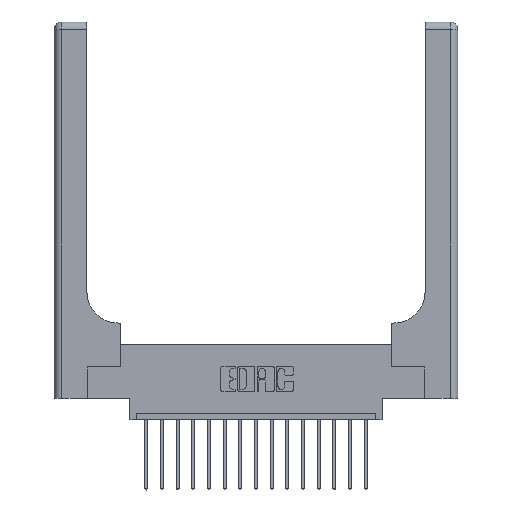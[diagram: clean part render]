
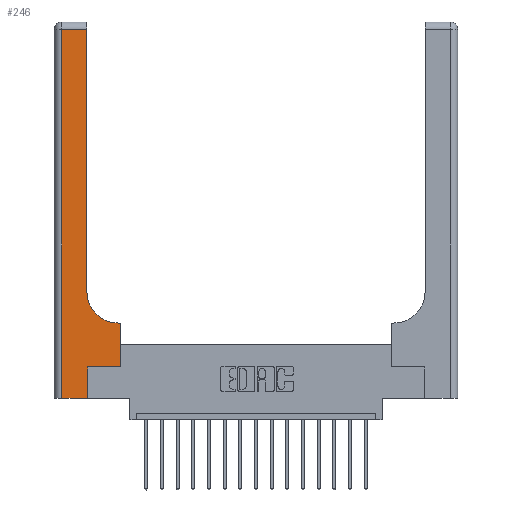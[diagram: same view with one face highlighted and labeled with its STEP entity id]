
A CAD part, top view. The second image highlights one B-rep face of the part: STEP entity #246.
In plain terms, the highlighted planar face has unit normal (0, 0, 1).
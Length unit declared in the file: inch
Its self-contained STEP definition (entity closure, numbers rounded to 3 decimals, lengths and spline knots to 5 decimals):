
#37 = EDGE_CURVE ( 'NONE', #4629, #17477, #10298, .T. ) ;
#77 = CARTESIAN_POINT ( 'NONE',  ( 0.06, 2.94, 0.37 ) ) ;
#246 = ADVANCED_FACE ( 'NONE', ( #18050 ), #10659, .F. ) ;
#384 = LINE ( 'NONE', #11235, #7409 ) ;
#398 = EDGE_CURVE ( 'NONE', #8279, #960, #17597, .T. ) ;
#650 = ORIENTED_EDGE ( 'NONE', *, *, #14773, .T. ) ;
#960 = VERTEX_POINT ( 'NONE', #5945 ) ;
#1144 = ORIENTED_EDGE ( 'NONE', *, *, #8607, .T. ) ;
#1529 = ORIENTED_EDGE ( 'NONE', *, *, #4312, .T. ) ;
#1647 = EDGE_LOOP ( 'NONE', ( #7086, #5595, #650, #1529, #4267, #12832, #17569, #1144, #8516 ) ) ;
#2311 = EDGE_CURVE ( 'NONE', #960, #9440, #13339, .T. ) ;
#2973 = LINE ( 'NONE', #3149, #10455 ) ;
#3149 = CARTESIAN_POINT ( 'NONE',  ( 0.265, 0., 0.37 ) ) ;
#3877 = LINE ( 'NONE', #10485, #13380 ) ;
#3951 = VERTEX_POINT ( 'NONE', #11939 ) ;
#4010 = AXIS2_PLACEMENT_3D ( 'NONE', #13622, #5151, #6574 ) ;
#4267 = ORIENTED_EDGE ( 'NONE', *, *, #10204, .T. ) ;
#4312 = EDGE_CURVE ( 'NONE', #15578, #3951, #3877, .T. ) ;
#4565 = CARTESIAN_POINT ( 'NONE',  ( 0.06, 3., 0.37 ) ) ;
#4629 = VERTEX_POINT ( 'NONE', #11442 ) ;
#4823 = EDGE_CURVE ( 'NONE', #9440, #11224, #384, .T. ) ;
#4839 = VECTOR ( 'NONE', #8584, 39.37008 ) ;
#5151 = DIRECTION ( 'NONE',  ( 0., 0., -1. ) ) ;
#5229 = EDGE_CURVE ( 'NONE', #17477, #16236, #8710, .T. ) ;
#5246 = CARTESIAN_POINT ( 'NONE',  ( 0.528, 0.25, 0.37 ) ) ;
#5595 = ORIENTED_EDGE ( 'NONE', *, *, #4823, .T. ) ;
#5945 = CARTESIAN_POINT ( 'NONE',  ( 0.26, 0.85, 0.37 ) ) ;
#6333 = DIRECTION ( 'NONE',  ( -1., 0., 0. ) ) ;
#6574 = DIRECTION ( 'NONE',  ( 1., 0., 0. ) ) ;
#7086 = ORIENTED_EDGE ( 'NONE', *, *, #2311, .T. ) ;
#7409 = VECTOR ( 'NONE', #15653, 39.37008 ) ;
#8157 = DIRECTION ( 'NONE',  ( 0., 1., 0. ) ) ;
#8260 = CARTESIAN_POINT ( 'NONE',  ( 0.26, 2.94, 0.37 ) ) ;
#8279 = VERTEX_POINT ( 'NONE', #15106 ) ;
#8474 = DIRECTION ( 'NONE',  ( 1., 0., 0. ) ) ;
#8516 = ORIENTED_EDGE ( 'NONE', *, *, #398, .T. ) ;
#8584 = DIRECTION ( 'NONE',  ( -1., 0., 0. ) ) ;
#8607 = EDGE_CURVE ( 'NONE', #16236, #8279, #8621, .T. ) ;
#8621 = LINE ( 'NONE', #11454, #4839 ) ;
#8710 = LINE ( 'NONE', #16796, #14240 ) ;
#8719 = DIRECTION ( 'NONE',  ( 0., -1., 0. ) ) ;
#9440 = VERTEX_POINT ( 'NONE', #8260 ) ;
#10134 = DIRECTION ( 'NONE',  ( 0., 1., 0. ) ) ;
#10204 = EDGE_CURVE ( 'NONE', #3951, #4629, #2973, .T. ) ;
#10298 = LINE ( 'NONE', #12775, #11617 ) ;
#10455 = VECTOR ( 'NONE', #14599, 39.37008 ) ;
#10485 = CARTESIAN_POINT ( 'NONE',  ( 0., 0., 0.37 ) ) ;
#10659 = PLANE ( 'NONE',  #16933 ) ;
#10673 = VECTOR ( 'NONE', #10134, 39.37008 ) ;
#11224 = VERTEX_POINT ( 'NONE', #77 ) ;
#11235 = CARTESIAN_POINT ( 'NONE',  ( 0., 2.94, 0.37 ) ) ;
#11442 = CARTESIAN_POINT ( 'NONE',  ( 0.265, 0.25, 0.37 ) ) ;
#11454 = CARTESIAN_POINT ( 'NONE',  ( 0.26, 0.6, 0.37 ) ) ;
#11617 = VECTOR ( 'NONE', #8474, 39.37008 ) ;
#11939 = CARTESIAN_POINT ( 'NONE',  ( 0.265, 0., 0.37 ) ) ;
#12058 = CARTESIAN_POINT ( 'NONE',  ( 0.528, 0.6, 0.37 ) ) ;
#12775 = CARTESIAN_POINT ( 'NONE',  ( 0.265, 0.25, 0.37 ) ) ;
#12832 = ORIENTED_EDGE ( 'NONE', *, *, #37, .T. ) ;
#13339 = LINE ( 'NONE', #15887, #10673 ) ;
#13380 = VECTOR ( 'NONE', #14735, 39.37008 ) ;
#13500 = CARTESIAN_POINT ( 'NONE',  ( 0., 3., 0.37 ) ) ;
#13622 = CARTESIAN_POINT ( 'NONE',  ( 0.51, 0.85, 0.37 ) ) ;
#14240 = VECTOR ( 'NONE', #8157, 39.37008 ) ;
#14599 = DIRECTION ( 'NONE',  ( 0., 1., 0. ) ) ;
#14735 = DIRECTION ( 'NONE',  ( 1., 0., 0. ) ) ;
#14773 = EDGE_CURVE ( 'NONE', #11224, #15578, #15368, .T. ) ;
#15106 = CARTESIAN_POINT ( 'NONE',  ( 0.51, 0.6, 0.37 ) ) ;
#15368 = LINE ( 'NONE', #4565, #17813 ) ;
#15578 = VERTEX_POINT ( 'NONE', #18025 ) ;
#15653 = DIRECTION ( 'NONE',  ( -1., 0., 0. ) ) ;
#15887 = CARTESIAN_POINT ( 'NONE',  ( 0.26, 3., 0.37 ) ) ;
#16184 = DIRECTION ( 'NONE',  ( 0., 0., -1. ) ) ;
#16236 = VERTEX_POINT ( 'NONE', #12058 ) ;
#16796 = CARTESIAN_POINT ( 'NONE',  ( 0.528, 0.25, 0.37 ) ) ;
#16933 = AXIS2_PLACEMENT_3D ( 'NONE', #13500, #16184, #6333 ) ;
#17477 = VERTEX_POINT ( 'NONE', #5246 ) ;
#17569 = ORIENTED_EDGE ( 'NONE', *, *, #5229, .T. ) ;
#17597 = CIRCLE ( 'NONE', #4010, 0.25 ) ;
#17813 = VECTOR ( 'NONE', #8719, 39.37008 ) ;
#18025 = CARTESIAN_POINT ( 'NONE',  ( 0.06, 0., 0.37 ) ) ;
#18050 = FACE_OUTER_BOUND ( 'NONE', #1647, .T. ) ;
